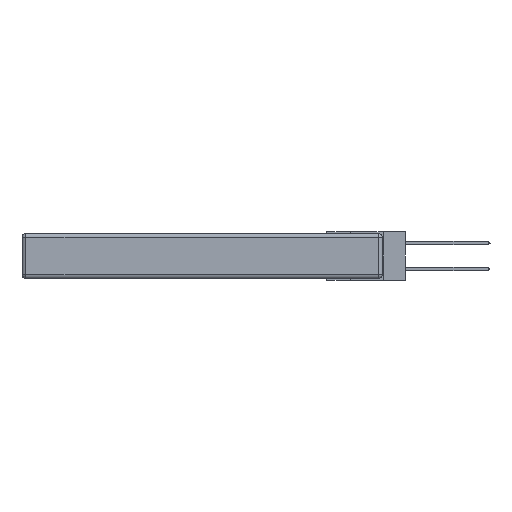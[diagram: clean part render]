
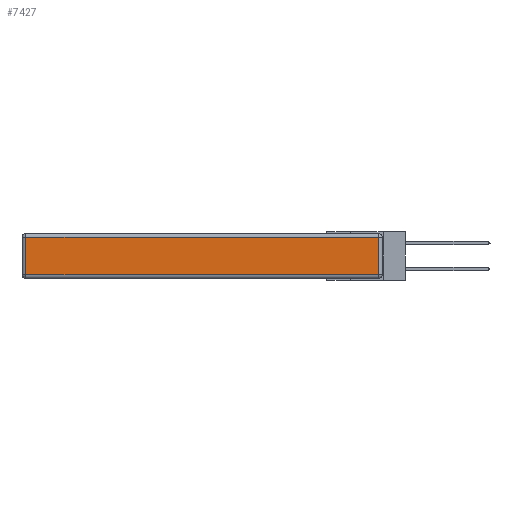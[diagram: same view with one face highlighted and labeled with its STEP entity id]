
A CAD part, left-side view. The second image highlights one B-rep face of the part: STEP entity #7427.
In plain terms, the highlighted planar face has unit normal (-1, 0, 0).
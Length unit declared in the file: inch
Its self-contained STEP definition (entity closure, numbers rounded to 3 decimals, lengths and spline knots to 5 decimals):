
#866 = EDGE_CURVE ( 'NONE', #31589, #21687, #12658, .T. ) ;
#1670 = EDGE_CURVE ( 'NONE', #21687, #18738, #3612, .T. ) ;
#2543 = VECTOR ( 'NONE', #14095, 39.37008 ) ;
#2564 = FACE_OUTER_BOUND ( 'NONE', #31878, .T. ) ;
#2704 = DIRECTION ( 'NONE',  ( 0., 1., 0. ) ) ;
#3612 = LINE ( 'NONE', #10839, #31956 ) ;
#3920 = CARTESIAN_POINT ( 'NONE',  ( 0., 0.03, -0.343 ) ) ;
#4186 = CARTESIAN_POINT ( 'NONE',  ( 0., 0., -0.343 ) ) ;
#4453 = LINE ( 'NONE', #7413, #18156 ) ;
#7413 = CARTESIAN_POINT ( 'NONE',  ( 0., 2.72, -0.343 ) ) ;
#7427 = ADVANCED_FACE ( 'NONE', ( #2564 ), #15448, .T. ) ;
#7906 = VERTEX_POINT ( 'NONE', #9547 ) ;
#9547 = CARTESIAN_POINT ( 'NONE',  ( 0., 2.72, -0.313 ) ) ;
#10839 = CARTESIAN_POINT ( 'NONE',  ( 0., 2.75, -0.03 ) ) ;
#12591 = DIRECTION ( 'NONE',  ( 0., 0., 1. ) ) ;
#12658 = LINE ( 'NONE', #3920, #18659 ) ;
#14095 = DIRECTION ( 'NONE',  ( 0., -1., 0. ) ) ;
#15216 = DIRECTION ( 'NONE',  ( 0., 0., -1. ) ) ;
#15448 = PLANE ( 'NONE',  #20875 ) ;
#15838 = CARTESIAN_POINT ( 'NONE',  ( 0., 0.03, -0.03 ) ) ;
#15932 = ORIENTED_EDGE ( 'NONE', *, *, #26850, .T. ) ;
#18156 = VECTOR ( 'NONE', #15216, 39.37008 ) ;
#18659 = VECTOR ( 'NONE', #28755, 39.37008 ) ;
#18738 = VERTEX_POINT ( 'NONE', #31265 ) ;
#20868 = ORIENTED_EDGE ( 'NONE', *, *, #866, .T. ) ;
#20875 = AXIS2_PLACEMENT_3D ( 'NONE', #4186, #34461, #12591 ) ;
#21405 = LINE ( 'NONE', #25253, #2543 ) ;
#21687 = VERTEX_POINT ( 'NONE', #15838 ) ;
#25253 = CARTESIAN_POINT ( 'NONE',  ( 0., 0., -0.313 ) ) ;
#26850 = EDGE_CURVE ( 'NONE', #18738, #7906, #4453, .T. ) ;
#28755 = DIRECTION ( 'NONE',  ( 0., 0., 1. ) ) ;
#28988 = ORIENTED_EDGE ( 'NONE', *, *, #1670, .T. ) ;
#30591 = CARTESIAN_POINT ( 'NONE',  ( 0., 0.03, -0.313 ) ) ;
#31265 = CARTESIAN_POINT ( 'NONE',  ( 0., 2.72, -0.03 ) ) ;
#31589 = VERTEX_POINT ( 'NONE', #30591 ) ;
#31878 = EDGE_LOOP ( 'NONE', ( #35455, #20868, #28988, #15932 ) ) ;
#31956 = VECTOR ( 'NONE', #2704, 39.37008 ) ;
#33586 = EDGE_CURVE ( 'NONE', #7906, #31589, #21405, .T. ) ;
#34461 = DIRECTION ( 'NONE',  ( -1., 0., 0. ) ) ;
#35455 = ORIENTED_EDGE ( 'NONE', *, *, #33586, .T. ) ;
